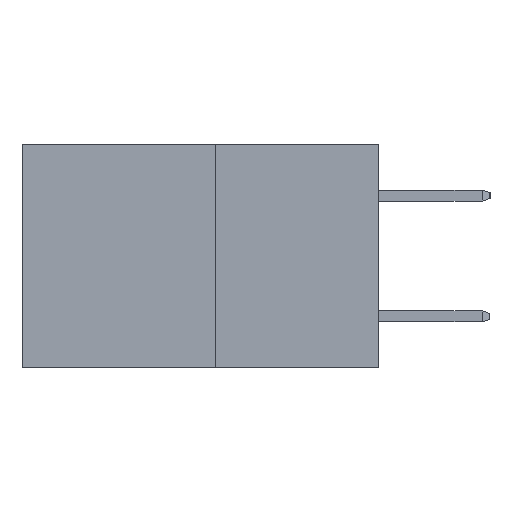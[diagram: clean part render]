
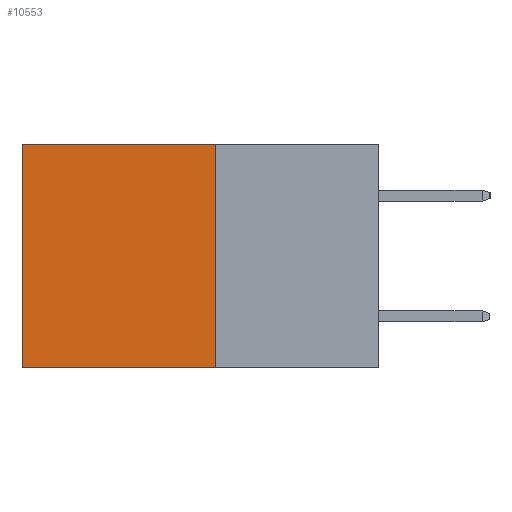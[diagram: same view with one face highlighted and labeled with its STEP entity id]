
A CAD part, left-side view. The second image highlights one B-rep face of the part: STEP entity #10553.
In plain terms, the highlighted planar face has unit normal (-1, 0, 0).
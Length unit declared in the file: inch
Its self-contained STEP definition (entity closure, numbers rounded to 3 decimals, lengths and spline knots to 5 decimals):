
#271 = ORIENTED_EDGE ( 'NONE', *, *, #15671, .T. ) ;
#529 = VECTOR ( 'NONE', #7751, 39.37008 ) ;
#1181 = CARTESIAN_POINT ( 'NONE',  ( 0.277, 0.27, -0.37 ) ) ;
#2501 = EDGE_LOOP ( 'NONE', ( #18345, #14991, #15450, #271 ) ) ;
#2707 = DIRECTION ( 'NONE',  ( 1., 0., 0. ) ) ;
#3923 = DIRECTION ( 'NONE',  ( 0., 0., -1. ) ) ;
#4288 = VECTOR ( 'NONE', #7082, 39.37008 ) ;
#4327 = VECTOR ( 'NONE', #3923, 39.37008 ) ;
#4531 = LINE ( 'NONE', #4817, #529 ) ;
#4817 = CARTESIAN_POINT ( 'NONE',  ( 0.277, 0.59, -0.37 ) ) ;
#4990 = VERTEX_POINT ( 'NONE', #5980 ) ;
#5297 = LINE ( 'NONE', #16969, #4327 ) ;
#5900 = EDGE_CURVE ( 'NONE', #11785, #8614, #10044, .T. ) ;
#5980 = CARTESIAN_POINT ( 'NONE',  ( 0.277, 0.59, 0. ) ) ;
#6162 = DIRECTION ( 'NONE',  ( 0., 1., 0. ) ) ;
#6202 = CARTESIAN_POINT ( 'NONE',  ( 0.277, 0.27, -0.37 ) ) ;
#7082 = DIRECTION ( 'NONE',  ( 0., 1., 0. ) ) ;
#7751 = DIRECTION ( 'NONE',  ( 0., 0., -1. ) ) ;
#8119 = AXIS2_PLACEMENT_3D ( 'NONE', #1181, #2707, #12969 ) ;
#8614 = VERTEX_POINT ( 'NONE', #10744 ) ;
#10044 = LINE ( 'NONE', #6202, #16315 ) ;
#10055 = PLANE ( 'NONE',  #8119 ) ;
#10302 = FACE_OUTER_BOUND ( 'NONE', #2501, .T. ) ;
#10442 = EDGE_CURVE ( 'NONE', #16547, #11785, #5297, .T. ) ;
#10553 = ADVANCED_FACE ( 'NONE', ( #10302 ), #10055, .F. ) ;
#10744 = CARTESIAN_POINT ( 'NONE',  ( 0.277, 0.59, -0.37 ) ) ;
#11785 = VERTEX_POINT ( 'NONE', #16989 ) ;
#12071 = LINE ( 'NONE', #17168, #4288 ) ;
#12969 = DIRECTION ( 'NONE',  ( 0., 0., -1. ) ) ;
#14991 = ORIENTED_EDGE ( 'NONE', *, *, #5900, .F. ) ;
#15409 = EDGE_CURVE ( 'NONE', #4990, #8614, #4531, .T. ) ;
#15450 = ORIENTED_EDGE ( 'NONE', *, *, #10442, .F. ) ;
#15671 = EDGE_CURVE ( 'NONE', #16547, #4990, #12071, .T. ) ;
#15998 = CARTESIAN_POINT ( 'NONE',  ( 0.277, 0.27, 0. ) ) ;
#16315 = VECTOR ( 'NONE', #6162, 39.37008 ) ;
#16547 = VERTEX_POINT ( 'NONE', #15998 ) ;
#16969 = CARTESIAN_POINT ( 'NONE',  ( 0.277, 0.27, -0.37 ) ) ;
#16989 = CARTESIAN_POINT ( 'NONE',  ( 0.277, 0.27, -0.37 ) ) ;
#17168 = CARTESIAN_POINT ( 'NONE',  ( 0.277, 0.27, 0. ) ) ;
#18345 = ORIENTED_EDGE ( 'NONE', *, *, #15409, .T. ) ;
